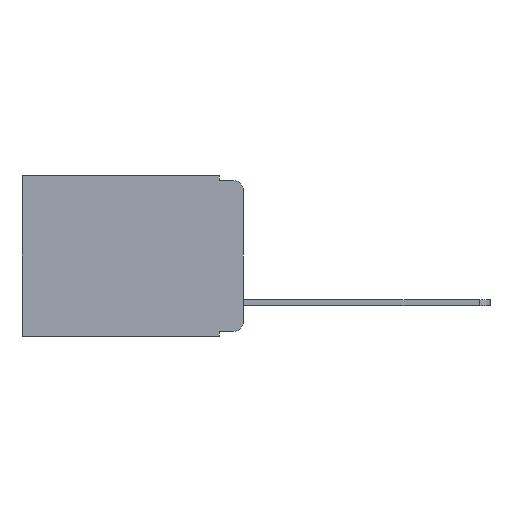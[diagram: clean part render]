
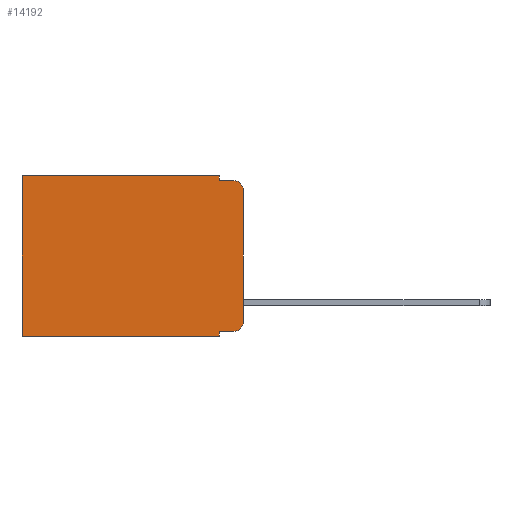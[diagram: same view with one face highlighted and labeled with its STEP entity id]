
A CAD part, left-side view. The second image highlights one B-rep face of the part: STEP entity #14192.
In plain terms, the highlighted planar face has unit normal (-1, 0, 0).
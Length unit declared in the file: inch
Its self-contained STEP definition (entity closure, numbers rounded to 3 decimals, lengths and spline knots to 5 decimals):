
#352 = CARTESIAN_POINT ( 'NONE',  ( 0.298, 0., 0. ) ) ;
#646 = CARTESIAN_POINT ( 'NONE',  ( 0.298, 0., -0.343 ) ) ;
#853 = EDGE_CURVE ( 'NONE', #2964, #1114, #9881, .T. ) ;
#855 = EDGE_CURVE ( 'NONE', #9024, #2964, #13332, .T. ) ;
#925 = CARTESIAN_POINT ( 'NONE',  ( 0.298, 0.051, -0.01 ) ) ;
#1114 = VERTEX_POINT ( 'NONE', #13077 ) ;
#1183 = PLANE ( 'NONE',  #6059 ) ;
#1241 = VERTEX_POINT ( 'NONE', #11767 ) ;
#2245 = LINE ( 'NONE', #7773, #12112 ) ;
#2392 = AXIS2_PLACEMENT_3D ( 'NONE', #12527, #4562, #13838 ) ;
#2675 = VECTOR ( 'NONE', #5917, 39.37008 ) ;
#2853 = CARTESIAN_POINT ( 'NONE',  ( 0.298, 0.051, -0.333 ) ) ;
#2870 = CIRCLE ( 'NONE', #12902, 0.02 ) ;
#2964 = VERTEX_POINT ( 'NONE', #10301 ) ;
#2970 = CARTESIAN_POINT ( 'NONE',  ( 0.298, 0.02, -0.01 ) ) ;
#2974 = LINE ( 'NONE', #646, #16111 ) ;
#3089 = EDGE_CURVE ( 'NONE', #9024, #8985, #2245, .T. ) ;
#3635 = VERTEX_POINT ( 'NONE', #10968 ) ;
#3986 = CARTESIAN_POINT ( 'NONE',  ( 0.298, 0., 0. ) ) ;
#4137 = EDGE_CURVE ( 'NONE', #14485, #9340, #2870, .T. ) ;
#4198 = CARTESIAN_POINT ( 'NONE',  ( 0.298, 0., 0. ) ) ;
#4323 = CARTESIAN_POINT ( 'NONE',  ( 0.298, 0.02, -0.333 ) ) ;
#4562 = DIRECTION ( 'NONE',  ( -1., 0., 0. ) ) ;
#4629 = CARTESIAN_POINT ( 'NONE',  ( 0.298, 0.051, -0.333 ) ) ;
#5341 = DIRECTION ( 'NONE',  ( 0., 0., -1. ) ) ;
#5844 = DIRECTION ( 'NONE',  ( 0., 0., -1. ) ) ;
#5917 = DIRECTION ( 'NONE',  ( 0., 0., -1. ) ) ;
#6018 = DIRECTION ( 'NONE',  ( 0., -1., 0. ) ) ;
#6059 = AXIS2_PLACEMENT_3D ( 'NONE', #3986, #13281, #5341 ) ;
#6182 = VECTOR ( 'NONE', #12978, 39.37008 ) ;
#6602 = LINE ( 'NONE', #11673, #6182 ) ;
#6707 = ORIENTED_EDGE ( 'NONE', *, *, #3089, .F. ) ;
#6759 = DIRECTION ( 'NONE',  ( 0., 0., -1. ) ) ;
#6961 = EDGE_CURVE ( 'NONE', #7514, #1241, #13836, .T. ) ;
#7115 = ORIENTED_EDGE ( 'NONE', *, *, #855, .T. ) ;
#7158 = ORIENTED_EDGE ( 'NONE', *, *, #8363, .F. ) ;
#7178 = ORIENTED_EDGE ( 'NONE', *, *, #853, .T. ) ;
#7369 = ORIENTED_EDGE ( 'NONE', *, *, #7516, .F. ) ;
#7514 = VERTEX_POINT ( 'NONE', #4323 ) ;
#7516 = EDGE_CURVE ( 'NONE', #16296, #3635, #14784, .T. ) ;
#7773 = CARTESIAN_POINT ( 'NONE',  ( 0.298, 0.051, 0. ) ) ;
#7824 = ORIENTED_EDGE ( 'NONE', *, *, #14001, .T. ) ;
#8238 = ORIENTED_EDGE ( 'NONE', *, *, #6961, .T. ) ;
#8363 = EDGE_CURVE ( 'NONE', #3635, #1114, #2974, .T. ) ;
#8407 = DIRECTION ( 'NONE',  ( 0., 0., -1. ) ) ;
#8985 = VERTEX_POINT ( 'NONE', #925 ) ;
#9024 = VERTEX_POINT ( 'NONE', #14328 ) ;
#9241 = LINE ( 'NONE', #352, #12299 ) ;
#9340 = VERTEX_POINT ( 'NONE', #2970 ) ;
#9881 = LINE ( 'NONE', #10465, #2675 ) ;
#9964 = LINE ( 'NONE', #4629, #16725 ) ;
#10301 = CARTESIAN_POINT ( 'NONE',  ( 0.298, 0.473, 0. ) ) ;
#10465 = CARTESIAN_POINT ( 'NONE',  ( 0.298, 0.473, 0. ) ) ;
#10538 = EDGE_CURVE ( 'NONE', #14485, #1241, #9241, .T. ) ;
#10786 = ORIENTED_EDGE ( 'NONE', *, *, #4137, .T. ) ;
#10968 = CARTESIAN_POINT ( 'NONE',  ( 0.298, 0.051, -0.343 ) ) ;
#10982 = CARTESIAN_POINT ( 'NONE',  ( 0.298, 0.051, 0. ) ) ;
#11031 = ORIENTED_EDGE ( 'NONE', *, *, #14624, .F. ) ;
#11673 = CARTESIAN_POINT ( 'NONE',  ( 0.298, 0.051, -0.01 ) ) ;
#11679 = CARTESIAN_POINT ( 'NONE',  ( 0.298, 0.02, -0.03 ) ) ;
#11767 = CARTESIAN_POINT ( 'NONE',  ( 0.298, 0., -0.313 ) ) ;
#11787 = VECTOR ( 'NONE', #8407, 39.37008 ) ;
#11809 = DIRECTION ( 'NONE',  ( -1., 0., 0. ) ) ;
#12112 = VECTOR ( 'NONE', #16061, 39.37008 ) ;
#12299 = VECTOR ( 'NONE', #5844, 39.37008 ) ;
#12527 = CARTESIAN_POINT ( 'NONE',  ( 0.298, 0.02, -0.313 ) ) ;
#12902 = AXIS2_PLACEMENT_3D ( 'NONE', #11679, #11809, #6759 ) ;
#12925 = VECTOR ( 'NONE', #16872, 39.37008 ) ;
#12978 = DIRECTION ( 'NONE',  ( 0., -1., 0. ) ) ;
#13077 = CARTESIAN_POINT ( 'NONE',  ( 0.298, 0.473, -0.343 ) ) ;
#13192 = ORIENTED_EDGE ( 'NONE', *, *, #10538, .F. ) ;
#13281 = DIRECTION ( 'NONE',  ( 1., 0., 0. ) ) ;
#13332 = LINE ( 'NONE', #4198, #12925 ) ;
#13836 = CIRCLE ( 'NONE', #2392, 0.02 ) ;
#13838 = DIRECTION ( 'NONE',  ( 0., 0., -1. ) ) ;
#14001 = EDGE_CURVE ( 'NONE', #16296, #7514, #9964, .T. ) ;
#14192 = ADVANCED_FACE ( 'NONE', ( #16918 ), #1183, .F. ) ;
#14328 = CARTESIAN_POINT ( 'NONE',  ( 0.298, 0.051, 0. ) ) ;
#14485 = VERTEX_POINT ( 'NONE', #15181 ) ;
#14624 = EDGE_CURVE ( 'NONE', #8985, #9340, #6602, .T. ) ;
#14784 = LINE ( 'NONE', #10982, #11787 ) ;
#15181 = CARTESIAN_POINT ( 'NONE',  ( 0.298, 0., -0.03 ) ) ;
#15251 = DIRECTION ( 'NONE',  ( 0., 1., 0. ) ) ;
#16061 = DIRECTION ( 'NONE',  ( 0., 0., -1. ) ) ;
#16111 = VECTOR ( 'NONE', #15251, 39.37008 ) ;
#16296 = VERTEX_POINT ( 'NONE', #2853 ) ;
#16361 = EDGE_LOOP ( 'NONE', ( #13192, #10786, #11031, #6707, #7115, #7178, #7158, #7369, #7824, #8238 ) ) ;
#16725 = VECTOR ( 'NONE', #6018, 39.37008 ) ;
#16872 = DIRECTION ( 'NONE',  ( 0., 1., 0. ) ) ;
#16918 = FACE_OUTER_BOUND ( 'NONE', #16361, .T. ) ;
